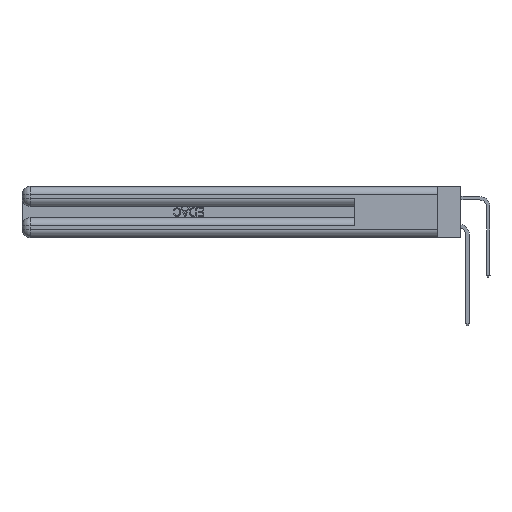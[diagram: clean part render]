
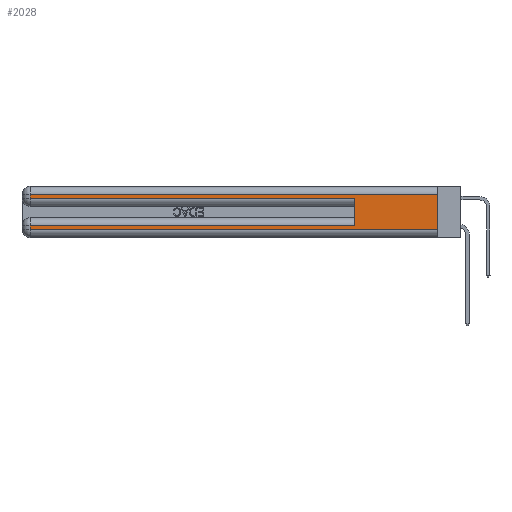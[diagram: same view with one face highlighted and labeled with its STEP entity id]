
A CAD part, left-side view. The second image highlights one B-rep face of the part: STEP entity #2028.
In plain terms, the highlighted planar face has unit normal (-1, 0, 0).
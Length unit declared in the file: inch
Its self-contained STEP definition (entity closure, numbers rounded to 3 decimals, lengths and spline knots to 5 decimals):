
#836 = CARTESIAN_POINT ( 'NONE',  ( 0., 2.94, 0.06 ) ) ;
#1302 = CARTESIAN_POINT ( 'NONE',  ( 0., 0., 0.285 ) ) ;
#2028 = ADVANCED_FACE ( 'NONE', ( #15786 ), #27284, .F. ) ;
#3716 = ORIENTED_EDGE ( 'NONE', *, *, #40919, .T. ) ;
#4195 = CARTESIAN_POINT ( 'NONE',  ( 0., 0., 0.37 ) ) ;
#4574 = VECTOR ( 'NONE', #21051, 39.37008 ) ;
#6773 = CARTESIAN_POINT ( 'NONE',  ( 0., 0., 0.06 ) ) ;
#6975 = CARTESIAN_POINT ( 'NONE',  ( 0., 0., 0.085 ) ) ;
#7135 = CARTESIAN_POINT ( 'NONE',  ( 0., 0., 0.37 ) ) ;
#7504 = DIRECTION ( 'NONE',  ( 1., 0., 0. ) ) ;
#7844 = ORIENTED_EDGE ( 'NONE', *, *, #41725, .T. ) ;
#8145 = VERTEX_POINT ( 'NONE', #11621 ) ;
#8488 = CARTESIAN_POINT ( 'NONE',  ( 0., 0.6, 0.285 ) ) ;
#9162 = EDGE_CURVE ( 'NONE', #30403, #37802, #37986, .T. ) ;
#10129 = DIRECTION ( 'NONE',  ( 0., 1., 0. ) ) ;
#10263 = DIRECTION ( 'NONE',  ( 0., 1., 0. ) ) ;
#10652 = EDGE_CURVE ( 'NONE', #14968, #18551, #26080, .T. ) ;
#11621 = CARTESIAN_POINT ( 'NONE',  ( 0., 2.94, 0.31 ) ) ;
#12766 = DIRECTION ( 'NONE',  ( 0., 0., -1. ) ) ;
#13106 = VERTEX_POINT ( 'NONE', #836 ) ;
#14235 = EDGE_CURVE ( 'NONE', #36270, #13106, #29473, .T. ) ;
#14968 = VERTEX_POINT ( 'NONE', #18947 ) ;
#15786 = FACE_OUTER_BOUND ( 'NONE', #22161, .T. ) ;
#17691 = CARTESIAN_POINT ( 'NONE',  ( 0., 0., 0.06 ) ) ;
#18551 = VERTEX_POINT ( 'NONE', #8488 ) ;
#18846 = CARTESIAN_POINT ( 'NONE',  ( 0., 2.94, 0.37 ) ) ;
#18947 = CARTESIAN_POINT ( 'NONE',  ( 0., 2.94, 0.285 ) ) ;
#19152 = CARTESIAN_POINT ( 'NONE',  ( 0., 2.94, 0.085 ) ) ;
#20158 = CARTESIAN_POINT ( 'NONE',  ( 0., 0., 0.31 ) ) ;
#21051 = DIRECTION ( 'NONE',  ( 0., -1., 0. ) ) ;
#21782 = CARTESIAN_POINT ( 'NONE',  ( 0., 0.6, 0.145 ) ) ;
#21985 = LINE ( 'NONE', #6975, #38364 ) ;
#22161 = EDGE_LOOP ( 'NONE', ( #26953, #28979, #3716, #39716, #23389, #7844, #42178, #27913 ) ) ;
#23389 = ORIENTED_EDGE ( 'NONE', *, *, #40916, .F. ) ;
#24008 = CARTESIAN_POINT ( 'NONE',  ( 0., 0., 0.31 ) ) ;
#24716 = AXIS2_PLACEMENT_3D ( 'NONE', #4195, #7504, #30540 ) ;
#26080 = LINE ( 'NONE', #1302, #41388 ) ;
#26089 = VERTEX_POINT ( 'NONE', #29180 ) ;
#26953 = ORIENTED_EDGE ( 'NONE', *, *, #9162, .F. ) ;
#27284 = PLANE ( 'NONE',  #24716 ) ;
#27698 = VECTOR ( 'NONE', #41341, 39.37008 ) ;
#27913 = ORIENTED_EDGE ( 'NONE', *, *, #39522, .T. ) ;
#28455 = VECTOR ( 'NONE', #35176, 39.37008 ) ;
#28647 = CARTESIAN_POINT ( 'NONE',  ( 0., 2.94, 0.37 ) ) ;
#28714 = LINE ( 'NONE', #28647, #35365 ) ;
#28979 = ORIENTED_EDGE ( 'NONE', *, *, #37249, .T. ) ;
#29180 = CARTESIAN_POINT ( 'NONE',  ( 0., 0.6, 0.085 ) ) ;
#29473 = LINE ( 'NONE', #18846, #28455 ) ;
#30165 = DIRECTION ( 'NONE',  ( 0., 0., -1. ) ) ;
#30286 = VECTOR ( 'NONE', #30165, 39.37008 ) ;
#30403 = VERTEX_POINT ( 'NONE', #24008 ) ;
#30540 = DIRECTION ( 'NONE',  ( 0., 0., -1. ) ) ;
#30873 = LINE ( 'NONE', #17691, #4574 ) ;
#35176 = DIRECTION ( 'NONE',  ( 0., 0., -1. ) ) ;
#35365 = VECTOR ( 'NONE', #12766, 39.37008 ) ;
#36270 = VERTEX_POINT ( 'NONE', #19152 ) ;
#36386 = LINE ( 'NONE', #21782, #27698 ) ;
#37249 = EDGE_CURVE ( 'NONE', #30403, #8145, #42222, .T. ) ;
#37802 = VERTEX_POINT ( 'NONE', #6773 ) ;
#37986 = LINE ( 'NONE', #7135, #30286 ) ;
#38364 = VECTOR ( 'NONE', #10263, 39.37008 ) ;
#39522 = EDGE_CURVE ( 'NONE', #13106, #37802, #30873, .T. ) ;
#39716 = ORIENTED_EDGE ( 'NONE', *, *, #10652, .T. ) ;
#40524 = DIRECTION ( 'NONE',  ( 0., -1., 0. ) ) ;
#40916 = EDGE_CURVE ( 'NONE', #26089, #18551, #36386, .T. ) ;
#40919 = EDGE_CURVE ( 'NONE', #8145, #14968, #28714, .T. ) ;
#41208 = VECTOR ( 'NONE', #10129, 39.37008 ) ;
#41341 = DIRECTION ( 'NONE',  ( 0., 0., 1. ) ) ;
#41388 = VECTOR ( 'NONE', #40524, 39.37008 ) ;
#41725 = EDGE_CURVE ( 'NONE', #26089, #36270, #21985, .T. ) ;
#42178 = ORIENTED_EDGE ( 'NONE', *, *, #14235, .T. ) ;
#42222 = LINE ( 'NONE', #20158, #41208 ) ;
